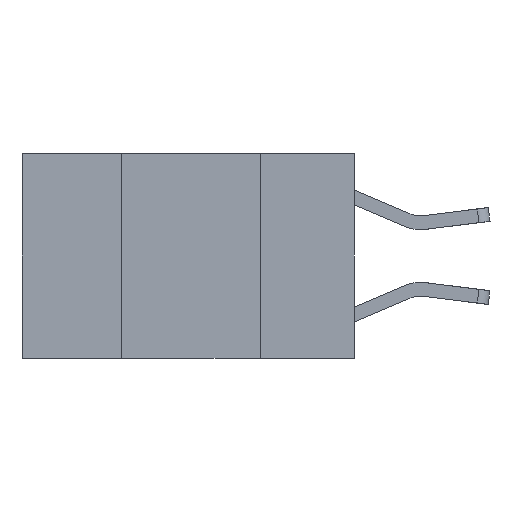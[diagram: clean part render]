
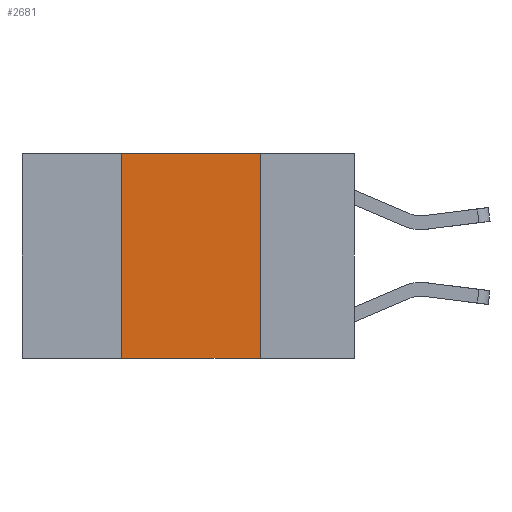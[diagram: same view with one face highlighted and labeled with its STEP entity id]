
A CAD part, left-side view. The second image highlights one B-rep face of the part: STEP entity #2681.
In plain terms, the highlighted planar face has unit normal (-1, 0, 0).
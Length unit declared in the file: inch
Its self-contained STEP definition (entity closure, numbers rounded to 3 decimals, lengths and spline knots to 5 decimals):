
#1468 = ORIENTED_EDGE ( 'NONE', *, *, #5383, .T. ) ;
#1648 = CARTESIAN_POINT ( 'NONE',  ( 0., 0.6, -0.37 ) ) ;
#1875 = FACE_OUTER_BOUND ( 'NONE', #4026, .T. ) ;
#2152 = DIRECTION ( 'NONE',  ( 0., 0., -1. ) ) ;
#2210 = VECTOR ( 'NONE', #3276, 39.37008 ) ;
#2681 = ADVANCED_FACE ( 'NONE', ( #1875 ), #6747, .F. ) ;
#3012 = CARTESIAN_POINT ( 'NONE',  ( 0., 0.42, 0. ) ) ;
#3088 = VECTOR ( 'NONE', #2152, 39.37008 ) ;
#3276 = DIRECTION ( 'NONE',  ( 0., -1., 0. ) ) ;
#3342 = VECTOR ( 'NONE', #7712, 39.37008 ) ;
#3419 = LINE ( 'NONE', #1648, #4847 ) ;
#3969 = DIRECTION ( 'NONE',  ( 1., 0., 0. ) ) ;
#4026 = EDGE_LOOP ( 'NONE', ( #5822, #8052, #7565, #1468 ) ) ;
#4191 = CARTESIAN_POINT ( 'NONE',  ( 0., 0.6, 0. ) ) ;
#4476 = AXIS2_PLACEMENT_3D ( 'NONE', #7234, #3969, #9219 ) ;
#4847 = VECTOR ( 'NONE', #7960, 39.37008 ) ;
#4997 = LINE ( 'NONE', #4191, #2210 ) ;
#5041 = VERTEX_POINT ( 'NONE', #3012 ) ;
#5188 = EDGE_CURVE ( 'NONE', #5041, #8469, #4997, .T. ) ;
#5383 = EDGE_CURVE ( 'NONE', #6595, #6874, #3419, .T. ) ;
#5578 = LINE ( 'NONE', #8443, #3088 ) ;
#5822 = ORIENTED_EDGE ( 'NONE', *, *, #5863, .F. ) ;
#5863 = EDGE_CURVE ( 'NONE', #8469, #6874, #5578, .T. ) ;
#6595 = VERTEX_POINT ( 'NONE', #9021 ) ;
#6676 = CARTESIAN_POINT ( 'NONE',  ( 0., 0.17, -0.37 ) ) ;
#6747 = PLANE ( 'NONE',  #4476 ) ;
#6828 = CARTESIAN_POINT ( 'NONE',  ( 0., 0.42, 0. ) ) ;
#6874 = VERTEX_POINT ( 'NONE', #6676 ) ;
#7234 = CARTESIAN_POINT ( 'NONE',  ( 0., 0.6, 0. ) ) ;
#7565 = ORIENTED_EDGE ( 'NONE', *, *, #9097, .F. ) ;
#7712 = DIRECTION ( 'NONE',  ( 0., 0., 1. ) ) ;
#7960 = DIRECTION ( 'NONE',  ( 0., -1., 0. ) ) ;
#8052 = ORIENTED_EDGE ( 'NONE', *, *, #5188, .F. ) ;
#8443 = CARTESIAN_POINT ( 'NONE',  ( 0., 0.17, 0. ) ) ;
#8469 = VERTEX_POINT ( 'NONE', #10612 ) ;
#9021 = CARTESIAN_POINT ( 'NONE',  ( 0., 0.42, -0.37 ) ) ;
#9097 = EDGE_CURVE ( 'NONE', #6595, #5041, #10282, .T. ) ;
#9219 = DIRECTION ( 'NONE',  ( 0., 0., -1. ) ) ;
#10282 = LINE ( 'NONE', #6828, #3342 ) ;
#10612 = CARTESIAN_POINT ( 'NONE',  ( 0., 0.17, 0. ) ) ;
